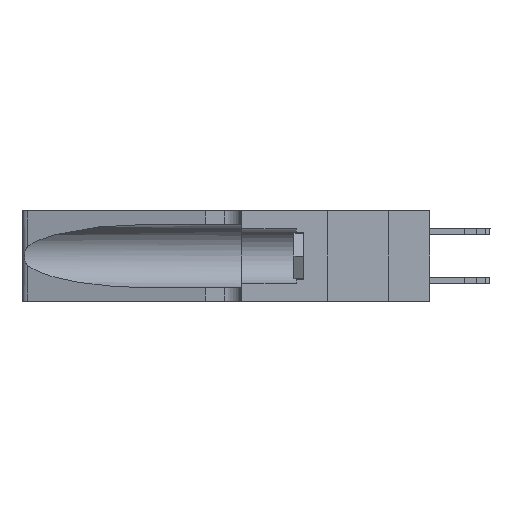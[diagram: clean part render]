
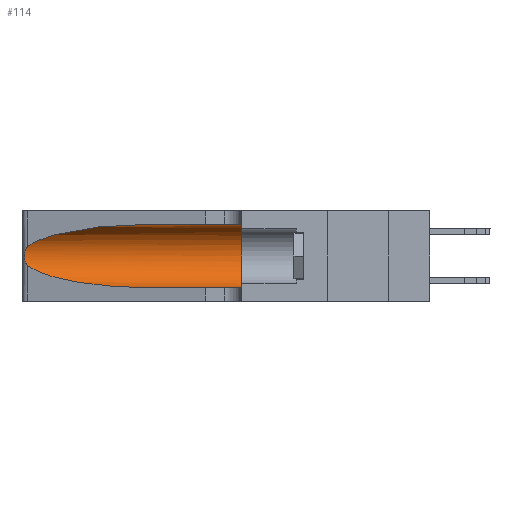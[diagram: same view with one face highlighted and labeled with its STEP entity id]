
A CAD part, left-side view. The second image highlights one B-rep face of the part: STEP entity #114.
In plain terms, the highlighted cylindrical face has radius 3.308 mm (diameter 6.617 mm), a partial arc.
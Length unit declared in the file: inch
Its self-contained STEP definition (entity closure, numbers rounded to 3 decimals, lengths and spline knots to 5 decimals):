
#114 = ADVANCED_FACE ( 'NONE', ( #25385 ), #13713, .F. ) ;
#227 = EDGE_CURVE ( 'NONE', #25943, #16219, #10861, .T. ) ;
#379 = CARTESIAN_POINT ( 'NONE',  ( 0.25639, 1.23184, 0.21858 ) ) ;
#466 = CARTESIAN_POINT ( 'NONE',  ( 0.25639, 1.23186, 0.15144 ) ) ;
#555 = CARTESIAN_POINT ( 'NONE',  ( 0.26017, 1.23833, 0.17102 ) ) ;
#788 = CARTESIAN_POINT ( 'NONE',  ( 0.1305, 1.61858, 0.05475 ) ) ;
#928 = CARTESIAN_POINT ( 'NONE',  ( 0.25555, 1.22993, 0.14849 ) ) ;
#1056 = LINE ( 'NONE', #19206, #16177 ) ;
#1184 = CARTESIAN_POINT ( 'NONE',  ( 0.25487, 1.22718, 0.14631 ) ) ;
#1353 = DIRECTION ( 'NONE',  ( 0., 1., 0. ) ) ;
#1387 = AXIS2_PLACEMENT_3D ( 'NONE', #19748, #1353, #19665 ) ;
#1508 = CARTESIAN_POINT ( 'NONE',  ( 0.2373, 1.15595, 0.08982 ) ) ;
#2245 = CIRCLE ( 'NONE', #1387, 0.13025 ) ;
#2504 = CARTESIAN_POINT ( 'NONE',  ( 0.26075, 1.23896, 0.19203 ) ) ;
#3172 = EDGE_CURVE ( 'NONE', #8435, #7545, #13981, .T. ) ;
#3254 = CARTESIAN_POINT ( 'NONE',  ( 0.2373, 1.15595, 0.28018 ) ) ;
#6698 = CARTESIAN_POINT ( 'NONE',  ( 0.26018, 1.23835, 0.19895 ) ) ;
#6885 = CARTESIAN_POINT ( 'NONE',  ( 0.25487, 1.22718, 0.14631 ) ) ;
#6970 = EDGE_CURVE ( 'NONE', #8338, #25943, #24415, .T. ) ;
#7037 = VECTOR ( 'NONE', #19389, 39.37008 ) ;
#7039 = CARTESIAN_POINT ( 'NONE',  ( 0.25487, 1.22718, 0.22369 ) ) ;
#7521 = ORIENTED_EDGE ( 'NONE', *, *, #3172, .T. ) ;
#7545 = VERTEX_POINT ( 'NONE', #10842 ) ;
#7708 = CARTESIAN_POINT ( 'NONE',  ( 0.25555, 1.22994, 0.2215 ) ) ;
#8338 = VERTEX_POINT ( 'NONE', #6885 ) ;
#8407 = EDGE_CURVE ( 'NONE', #8435, #25511, #1056, .T. ) ;
#8435 = VERTEX_POINT ( 'NONE', #25201 ) ;
#8762 = CARTESIAN_POINT ( 'NONE',  ( 0.25789, 1.23486, 0.15765 ) ) ;
#9563 = B_SPLINE_CURVE_WITH_KNOTS ( 'NONE', 3,
 ( #19810, #7708, #379, #20232, #18289, #6698, #2504, #18644, #555, #16680, #8762, #466, #928, #1184 ),
 .UNSPECIFIED., .F., .F.,
 ( 4, 2, 2, 2, 2, 2, 4 ),
 ( 0., 0.00027, 0.00053, 0.00107, 0.0016, 0.00187, 0.00214 ),
 .UNSPECIFIED. ) ;
#9605 = CARTESIAN_POINT ( 'NONE',  ( 0.18966, 0.96281, 0.05475 ) ) ;
#10842 = CARTESIAN_POINT ( 'NONE',  ( 0.25487, 1.22718, 0.22369 ) ) ;
#10861 = LINE ( 'NONE', #788, #7037 ) ;
#11196 = AXIS2_PLACEMENT_3D ( 'NONE', #15036, #11436, #23582 ) ;
#11436 = DIRECTION ( 'NONE',  ( 0., -1., 0. ) ) ;
#12796 = EDGE_CURVE ( 'NONE', #7545, #8338, #9563, .T. ) ;
#12889 = EDGE_LOOP ( 'NONE', ( #7521, #21257, #13011, #22257, #12929, #19677 ) ) ;
#12929 = ORIENTED_EDGE ( 'NONE', *, *, #20831, .F. ) ;
#13011 = ORIENTED_EDGE ( 'NONE', *, *, #6970, .T. ) ;
#13713 = CYLINDRICAL_SURFACE ( 'NONE', #11196, 0.13025 ) ;
#13981 =( BOUNDED_CURVE ( )  B_SPLINE_CURVE ( 3, ( #17117, #19151, #3254, #7039 ),
 .UNSPECIFIED., .F., .F. ) 
 B_SPLINE_CURVE_WITH_KNOTS ( ( 4, 4 ),
 ( 1.5708, 2.84003 ),
 .UNSPECIFIED. ) 
 CURVE ( )  GEOMETRIC_REPRESENTATION_ITEM ( )  RATIONAL_B_SPLINE_CURVE ( ( 1., 0.87, 0.87, 1. ) ) 
 REPRESENTATION_ITEM ( '' )  );
#15036 = CARTESIAN_POINT ( 'NONE',  ( 0.1305, 1.61858, 0.185 ) ) ;
#16177 = VECTOR ( 'NONE', #21056, 39.37008 ) ;
#16219 = VERTEX_POINT ( 'NONE', #19794 ) ;
#16667 = CARTESIAN_POINT ( 'NONE',  ( 0.1305, 0.72297, 0.05475 ) ) ;
#16680 = CARTESIAN_POINT ( 'NONE',  ( 0.25856, 1.23593, 0.16098 ) ) ;
#17117 = CARTESIAN_POINT ( 'NONE',  ( 0.1305, 0.72297, 0.31525 ) ) ;
#17437 = CARTESIAN_POINT ( 'NONE',  ( 0.25487, 1.22718, 0.14631 ) ) ;
#18289 = CARTESIAN_POINT ( 'NONE',  ( 0.25854, 1.2359, 0.20912 ) ) ;
#18644 = CARTESIAN_POINT ( 'NONE',  ( 0.26075, 1.23896, 0.178 ) ) ;
#19151 = CARTESIAN_POINT ( 'NONE',  ( 0.18966, 0.96281, 0.31525 ) ) ;
#19206 = CARTESIAN_POINT ( 'NONE',  ( 0.1305, 1.61858, 0.31525 ) ) ;
#19389 = DIRECTION ( 'NONE',  ( 0., -1., 0. ) ) ;
#19442 = CARTESIAN_POINT ( 'NONE',  ( 0.1305, 0.35, 0.31525 ) ) ;
#19665 = DIRECTION ( 'NONE',  ( 0., 0., 1. ) ) ;
#19677 = ORIENTED_EDGE ( 'NONE', *, *, #8407, .F. ) ;
#19748 = CARTESIAN_POINT ( 'NONE',  ( 0.1305, 0.35, 0.185 ) ) ;
#19794 = CARTESIAN_POINT ( 'NONE',  ( 0.1305, 0.35, 0.05475 ) ) ;
#19810 = CARTESIAN_POINT ( 'NONE',  ( 0.25487, 1.22718, 0.22369 ) ) ;
#20232 = CARTESIAN_POINT ( 'NONE',  ( 0.25787, 1.23484, 0.2124 ) ) ;
#20831 = EDGE_CURVE ( 'NONE', #25511, #16219, #2245, .T. ) ;
#21056 = DIRECTION ( 'NONE',  ( 0., -1., 0. ) ) ;
#21257 = ORIENTED_EDGE ( 'NONE', *, *, #12796, .T. ) ;
#22257 = ORIENTED_EDGE ( 'NONE', *, *, #227, .T. ) ;
#23582 = DIRECTION ( 'NONE',  ( 0., 0., -1. ) ) ;
#24415 =( BOUNDED_CURVE ( )  B_SPLINE_CURVE ( 3, ( #17437, #1508, #9605, #25718 ),
 .UNSPECIFIED., .F., .T. ) 
 B_SPLINE_CURVE_WITH_KNOTS ( ( 4, 4 ),
 ( 3.44316, 4.71239 ),
 .UNSPECIFIED. ) 
 CURVE ( )  GEOMETRIC_REPRESENTATION_ITEM ( )  RATIONAL_B_SPLINE_CURVE ( ( 1., 0.87, 0.87, 1. ) ) 
 REPRESENTATION_ITEM ( '' )  );
#25201 = CARTESIAN_POINT ( 'NONE',  ( 0.1305, 0.72297, 0.31525 ) ) ;
#25385 = FACE_OUTER_BOUND ( 'NONE', #12889, .T. ) ;
#25511 = VERTEX_POINT ( 'NONE', #19442 ) ;
#25718 = CARTESIAN_POINT ( 'NONE',  ( 0.1305, 0.72297, 0.05475 ) ) ;
#25943 = VERTEX_POINT ( 'NONE', #16667 ) ;
